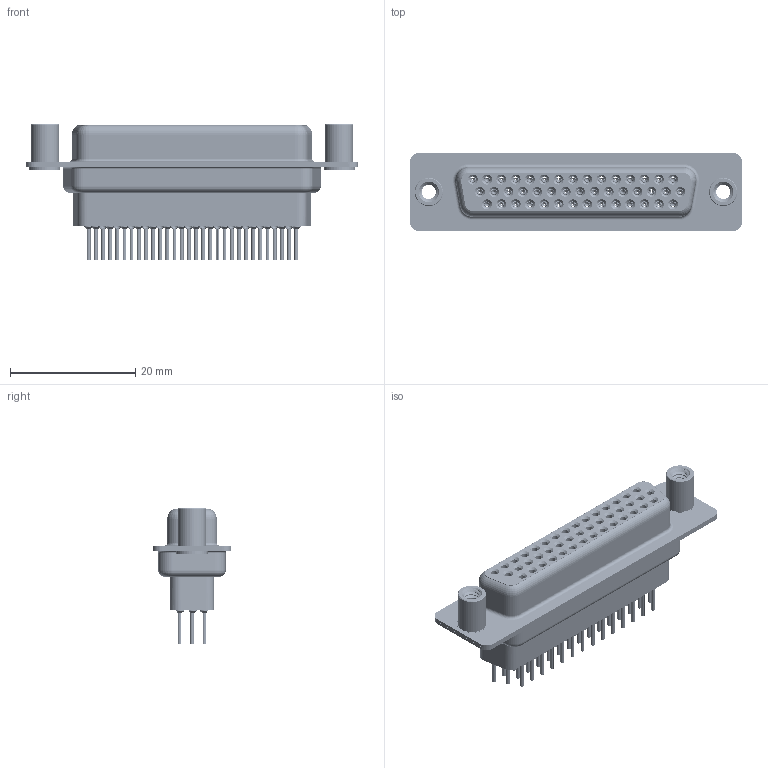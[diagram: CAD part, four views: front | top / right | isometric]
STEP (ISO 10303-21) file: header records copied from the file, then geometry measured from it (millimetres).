
FILE_DESCRIPTION (( 'STEP AP203' ), '1' );
FILE_NAME ('638-044-331-258.STEP', '2020-07-18T23:21:03', ( '' ), ( '' ), 'SwSTEP 2.0', 'SolidWorks 2020', '' );
FILE_SCHEMA (( 'CONFIG_CONTROL_DESIGN' ));
Length unit declared in the file: millimetre
Products named in the file (8): 638-044-331-258; 638 Shell Rear_44 Contacts; 638 Contact Row 3_31; 638 Shell Front_44 Contacts; 638 Contact Row 2_31; 638 Housing_44 Contacts HP; 638 4-40 Threaded Standoff; 638 Contact Row 1_31
Assembly tree (49 placements, depth 2):
  638-044-331-258
    638 Housing_44 Contacts HP
    638 Shell Front_44 Contacts
    638 Shell Rear_44 Contacts
    638 Contact Row 1_31  x15
    638 Contact Row 2_31  x15
    638 Contact Row 3_31  x14
    638 4-40 Threaded Standoff  x2
Bounding box: 53.04 x 12.6 x 21.7 mm (x, y, z)
Volume: 4046.1 mm3; surface area: 15545.1 mm2
Topology: 49 solids, 49 shells, 5725 faces, 14681 edges, 9155 vertices
Faces by surface type: cylinder 1617, plane 1433, torus 1113, bspline 886, cone 676
Entity records: 40493 total; most frequent: CARTESIAN_POINT 11184, DIRECTION 6048, ORIENTED_EDGE 5486, EDGE_CURVE 2743, AXIS2_PLACEMENT_3D 2543, VERTEX_POINT 1734, EDGE_LOOP 1409, CIRCLE 1389
